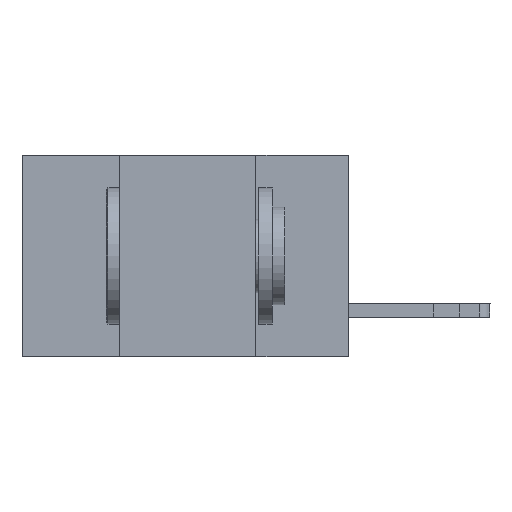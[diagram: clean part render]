
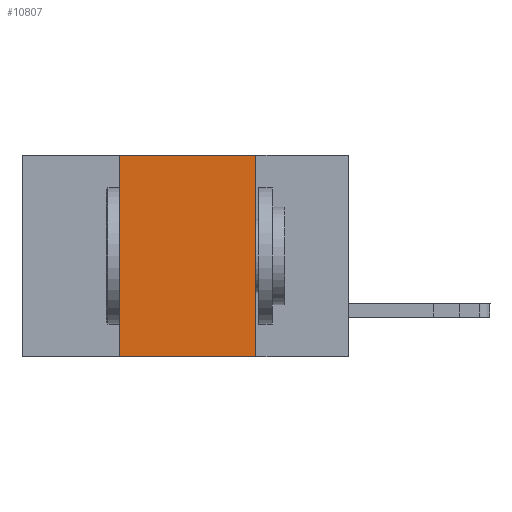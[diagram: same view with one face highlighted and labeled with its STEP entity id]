
A CAD part, left-side view. The second image highlights one B-rep face of the part: STEP entity #10807.
In plain terms, the highlighted planar face has unit normal (-1, 0, 0).
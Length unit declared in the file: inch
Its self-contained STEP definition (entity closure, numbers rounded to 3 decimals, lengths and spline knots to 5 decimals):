
#90 = EDGE_CURVE ( 'NONE', #6350, #10271, #7883, .T. ) ;
#158 = CARTESIAN_POINT ( 'NONE',  ( 0., 0.17, -0.37 ) ) ;
#426 = AXIS2_PLACEMENT_3D ( 'NONE', #1385, #3378, #8664 ) ;
#644 = EDGE_CURVE ( 'NONE', #727, #6350, #9887, .T. ) ;
#727 = VERTEX_POINT ( 'NONE', #5816 ) ;
#798 = VECTOR ( 'NONE', #7251, 39.37008 ) ;
#806 = LINE ( 'NONE', #8582, #4193 ) ;
#1385 = CARTESIAN_POINT ( 'NONE',  ( 0., 0.6, 0. ) ) ;
#1420 = DIRECTION ( 'NONE',  ( 0., 0., 1. ) ) ;
#1903 = CARTESIAN_POINT ( 'NONE',  ( 0., 0.42, 0. ) ) ;
#2040 = VERTEX_POINT ( 'NONE', #158 ) ;
#3102 = PLANE ( 'NONE',  #426 ) ;
#3204 = DIRECTION ( 'NONE',  ( 0., -1., 0. ) ) ;
#3378 = DIRECTION ( 'NONE',  ( 1., 0., 0. ) ) ;
#3459 = DIRECTION ( 'NONE',  ( 0., 0., -1. ) ) ;
#3651 = EDGE_CURVE ( 'NONE', #10271, #2040, #806, .T. ) ;
#3706 = ORIENTED_EDGE ( 'NONE', *, *, #6847, .T. ) ;
#3753 = ORIENTED_EDGE ( 'NONE', *, *, #3651, .F. ) ;
#3885 = VECTOR ( 'NONE', #1420, 39.37008 ) ;
#4193 = VECTOR ( 'NONE', #3459, 39.37008 ) ;
#5816 = CARTESIAN_POINT ( 'NONE',  ( 0., 0.42, -0.37 ) ) ;
#6350 = VERTEX_POINT ( 'NONE', #1903 ) ;
#6477 = FACE_OUTER_BOUND ( 'NONE', #9748, .T. ) ;
#6847 = EDGE_CURVE ( 'NONE', #727, #2040, #7958, .T. ) ;
#7251 = DIRECTION ( 'NONE',  ( 0., -1., 0. ) ) ;
#7883 = LINE ( 'NONE', #9896, #9046 ) ;
#7958 = LINE ( 'NONE', #9800, #798 ) ;
#8247 = CARTESIAN_POINT ( 'NONE',  ( 0., 0.17, 0. ) ) ;
#8397 = ORIENTED_EDGE ( 'NONE', *, *, #90, .F. ) ;
#8582 = CARTESIAN_POINT ( 'NONE',  ( 0., 0.17, -0.37 ) ) ;
#8664 = DIRECTION ( 'NONE',  ( 0., 0., -1. ) ) ;
#9045 = CARTESIAN_POINT ( 'NONE',  ( 0., 0.42, -0.37 ) ) ;
#9046 = VECTOR ( 'NONE', #3204, 39.37008 ) ;
#9748 = EDGE_LOOP ( 'NONE', ( #3753, #8397, #10805, #3706 ) ) ;
#9800 = CARTESIAN_POINT ( 'NONE',  ( 0., 0.6, -0.37 ) ) ;
#9887 = LINE ( 'NONE', #9045, #3885 ) ;
#9896 = CARTESIAN_POINT ( 'NONE',  ( 0., 0.6, 0. ) ) ;
#10271 = VERTEX_POINT ( 'NONE', #8247 ) ;
#10805 = ORIENTED_EDGE ( 'NONE', *, *, #644, .F. ) ;
#10807 = ADVANCED_FACE ( 'NONE', ( #6477 ), #3102, .F. ) ;
